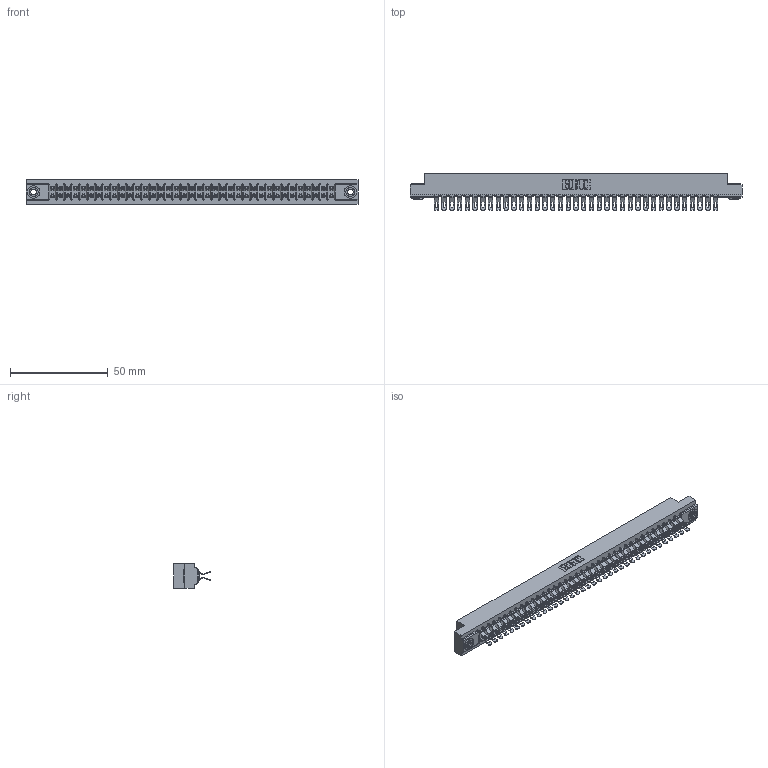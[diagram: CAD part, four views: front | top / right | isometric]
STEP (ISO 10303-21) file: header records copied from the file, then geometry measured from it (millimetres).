
FILE_DESCRIPTION (( 'STEP AP203' ), '1' );
FILE_NAME ('307-074-455-203.STEP', '2020-10-01T03:42:29', ( '' ), ( '' ), 'SwSTEP 2.0', 'SolidWorks 2020', '' );
FILE_SCHEMA (( 'CONFIG_CONTROL_DESIGN' ));
Length unit declared in the file: inch
Products named in the file (4): 307 Part_.156 Dia Mounting Holes; 345-250-002_345-250-002-102; 307-074-455-203; 307-290-001_555
Assembly tree (77 placements, depth 2):
  307-074-455-203
    307 Part_.156 Dia Mounting Holes
    307-290-001_555  x74
    345-250-002_345-250-002-102  x2
Bounding box: 169.62 x 18.75 x 12.7 mm (x, y, z)
Volume: 18223.6 mm3; surface area: 23670.8 mm2
Topology: 77 solids, 77 shells, 4722 faces, 13829 edges, 9014 vertices
Faces by surface type: plane 2610, cylinder 2028, sphere 76, cone 8
Entity records: 35122 total; most frequent: CARTESIAN_POINT 5734, ORIENTED_EDGE 5676, DIRECTION 5640, EDGE_CURVE 2838, VECTOR 2156, LINE 2156, VERTEX_POINT 1836, AXIS2_PLACEMENT_3D 1742
